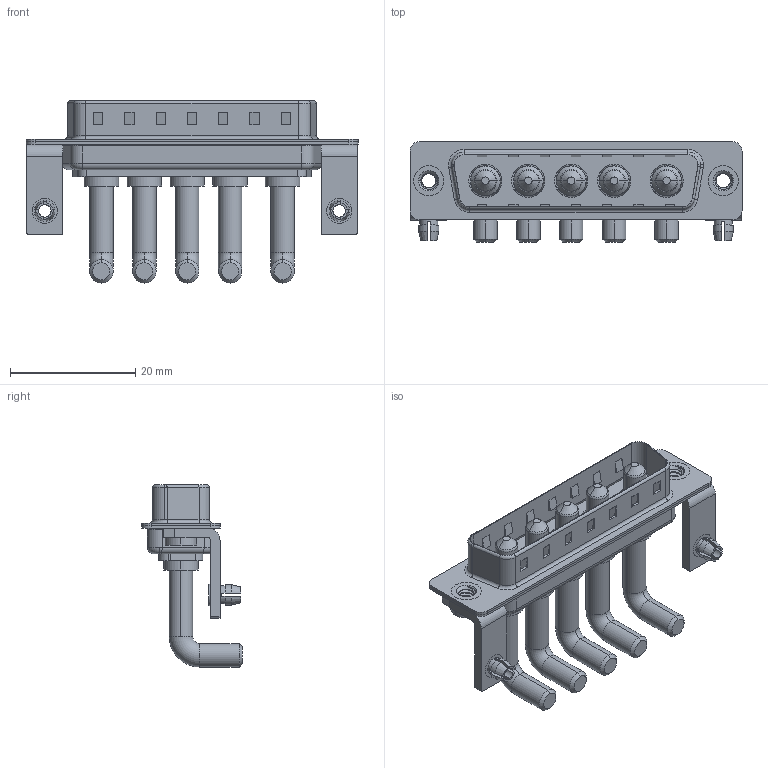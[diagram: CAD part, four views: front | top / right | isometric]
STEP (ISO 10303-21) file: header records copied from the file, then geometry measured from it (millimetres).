
FILE_DESCRIPTION (( 'STEP AP203' ), '1' );
FILE_NAME ('629-5W5-250-4NB.STEP', '2022-05-07T07:52:44', ( '' ), ( '' ), 'SwSTEP 2.0', 'SolidWorks 2020', '' );
FILE_SCHEMA (( 'CONFIG_CONTROL_DESIGN' ));
Length unit declared in the file: millimetre
Products named in the file (8): 629Combo Threaded Rivet_2; 629Combo Board Lock; 629Combo Shell Rear_25 Contacts; 629Combo Shell Front_25 Contacts; Power Pin_Ext 40A RA; 629Combo Stabilizer Bracket; 629-5W5-250-4NB; 629Combo Housing_5W5
Assembly tree (14 placements, depth 2):
  629-5W5-250-4NB
    629Combo Housing_5W5
    629Combo Shell Rear_25 Contacts
    629Combo Shell Front_25 Contacts
    629Combo Threaded Rivet_2  x2
    629Combo Stabilizer Bracket  x2
    629Combo Board Lock  x2
    Power Pin_Ext 40A RA  x5
Bounding box: 53.05 x 16.05 x 29.11 mm (x, y, z)
Volume: 4508.4 mm3; surface area: 8638.6 mm2
Topology: 19 solids, 19 shells, 731 faces, 1789 edges, 1126 vertices
Faces by surface type: cylinder 298, plane 289, torus 70, cone 63, bspline 11
Entity records: 16920 total; most frequent: CARTESIAN_POINT 4081, DIRECTION 2573, ORIENTED_EDGE 2400, EDGE_CURVE 1200, AXIS2_PLACEMENT_3D 943, VERTEX_POINT 760, VECTOR 687, LINE 687
